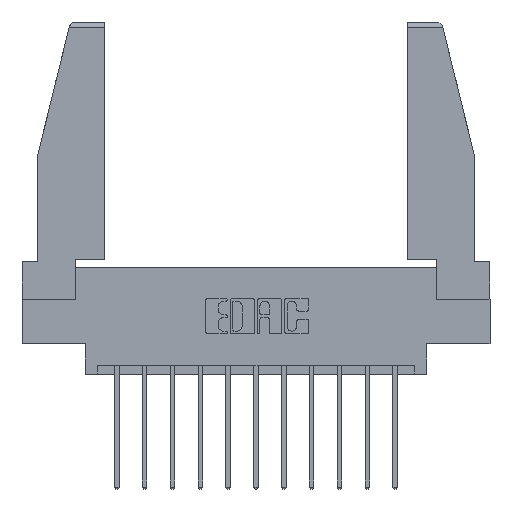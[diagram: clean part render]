
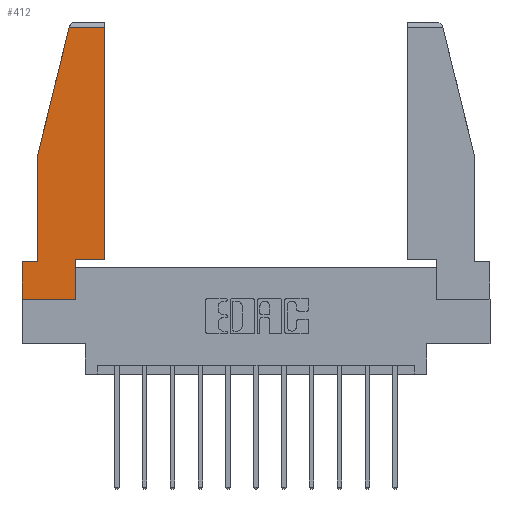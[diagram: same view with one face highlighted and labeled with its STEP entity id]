
A CAD part, top view. The second image highlights one B-rep face of the part: STEP entity #412.
In plain terms, the highlighted planar face has unit normal (0, 0, 1).
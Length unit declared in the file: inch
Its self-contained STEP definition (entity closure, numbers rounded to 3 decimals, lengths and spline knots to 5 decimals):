
#412 = ADVANCED_FACE ( 'NONE', ( #4987 ), #615, .T. ) ;
#585 = EDGE_CURVE ( 'NONE', #11403, #2946, #2954, .T. ) ;
#615 = PLANE ( 'NONE',  #14132 ) ;
#781 = VERTEX_POINT ( 'NONE', #3875 ) ;
#882 = CARTESIAN_POINT ( 'NONE',  ( 0.297, 0., 0. ) ) ;
#1013 = ORIENTED_EDGE ( 'NONE', *, *, #5995, .T. ) ;
#1213 = LINE ( 'NONE', #9749, #13338 ) ;
#1248 = LINE ( 'NONE', #13037, #14438 ) ;
#1389 = DIRECTION ( 'NONE',  ( 1., 0., 0. ) ) ;
#1553 = EDGE_CURVE ( 'NONE', #7797, #781, #8787, .T. ) ;
#1920 = CARTESIAN_POINT ( 'NONE',  ( 0.271, 1.55, 0. ) ) ;
#2297 = DIRECTION ( 'NONE',  ( 0., 1., 0. ) ) ;
#2397 = ORIENTED_EDGE ( 'NONE', *, *, #3390, .T. ) ;
#2586 = VECTOR ( 'NONE', #1389, 39.37008 ) ;
#2946 = VERTEX_POINT ( 'NONE', #5518 ) ;
#2954 = LINE ( 'NONE', #7276, #2586 ) ;
#2974 = DIRECTION ( 'NONE',  ( -0.239, -0.971, 0. ) ) ;
#3390 = EDGE_CURVE ( 'NONE', #13876, #11403, #7175, .T. ) ;
#3395 = VECTOR ( 'NONE', #9940, 39.37008 ) ;
#3468 = CARTESIAN_POINT ( 'NONE',  ( 0., 0., 0. ) ) ;
#3744 = EDGE_CURVE ( 'NONE', #781, #8341, #7984, .T. ) ;
#3875 = CARTESIAN_POINT ( 'NONE',  ( 0.086, 0.8, 0. ) ) ;
#3936 = LINE ( 'NONE', #5232, #12155 ) ;
#4003 = EDGE_CURVE ( 'NONE', #2946, #7961, #9413, .T. ) ;
#4074 = CARTESIAN_POINT ( 'NONE',  ( 0.086, 0.8, 0. ) ) ;
#4255 = CARTESIAN_POINT ( 'NONE',  ( 0., 0., 0. ) ) ;
#4987 = FACE_OUTER_BOUND ( 'NONE', #12241, .T. ) ;
#5231 = ORIENTED_EDGE ( 'NONE', *, *, #1553, .T. ) ;
#5232 = CARTESIAN_POINT ( 'NONE',  ( 0., 1.52, 0. ) ) ;
#5275 = DIRECTION ( 'NONE',  ( 1., 0., 0. ) ) ;
#5518 = CARTESIAN_POINT ( 'NONE',  ( 0.461, 0.223, 0. ) ) ;
#5841 = CARTESIAN_POINT ( 'NONE',  ( 0.297, 0.223, 0. ) ) ;
#5995 = EDGE_CURVE ( 'NONE', #8341, #9456, #1248, .T. ) ;
#6191 = ORIENTED_EDGE ( 'NONE', *, *, #4003, .T. ) ;
#6343 = CARTESIAN_POINT ( 'NONE',  ( 0., 0., 0. ) ) ;
#6649 = DIRECTION ( 'NONE',  ( 0., 1., 0. ) ) ;
#7175 = LINE ( 'NONE', #882, #9466 ) ;
#7276 = CARTESIAN_POINT ( 'NONE',  ( 0.297, 0.223, 0. ) ) ;
#7795 = DIRECTION ( 'NONE',  ( 1., 0., 0. ) ) ;
#7797 = VERTEX_POINT ( 'NONE', #11189 ) ;
#7961 = VERTEX_POINT ( 'NONE', #13493 ) ;
#7984 = LINE ( 'NONE', #4074, #3395 ) ;
#8187 = ORIENTED_EDGE ( 'NONE', *, *, #9567, .T. ) ;
#8341 = VERTEX_POINT ( 'NONE', #11113 ) ;
#8418 = ORIENTED_EDGE ( 'NONE', *, *, #3744, .T. ) ;
#8441 = DIRECTION ( 'NONE',  ( 0., -1., 0. ) ) ;
#8645 = ORIENTED_EDGE ( 'NONE', *, *, #585, .T. ) ;
#8787 = LINE ( 'NONE', #1920, #13576 ) ;
#9253 = CARTESIAN_POINT ( 'NONE',  ( 0.461, 0.223, 0. ) ) ;
#9347 = EDGE_CURVE ( 'NONE', #9456, #11376, #1213, .T. ) ;
#9413 = LINE ( 'NONE', #9253, #15070 ) ;
#9456 = VERTEX_POINT ( 'NONE', #10641 ) ;
#9466 = VECTOR ( 'NONE', #6649, 39.37008 ) ;
#9567 = EDGE_CURVE ( 'NONE', #7961, #7797, #3936, .T. ) ;
#9711 = VECTOR ( 'NONE', #5275, 39.37008 ) ;
#9749 = CARTESIAN_POINT ( 'NONE',  ( 0., 0.21, 0. ) ) ;
#9940 = DIRECTION ( 'NONE',  ( 0., -1., 0. ) ) ;
#10641 = CARTESIAN_POINT ( 'NONE',  ( 0., 0.21, 0. ) ) ;
#10754 = ORIENTED_EDGE ( 'NONE', *, *, #9347, .T. ) ;
#11113 = CARTESIAN_POINT ( 'NONE',  ( 0.086, 0.21, 0. ) ) ;
#11189 = CARTESIAN_POINT ( 'NONE',  ( 0.2636, 1.52, 0. ) ) ;
#11339 = ORIENTED_EDGE ( 'NONE', *, *, #13700, .T. ) ;
#11376 = VERTEX_POINT ( 'NONE', #3468 ) ;
#11403 = VERTEX_POINT ( 'NONE', #5841 ) ;
#11758 = DIRECTION ( 'NONE',  ( -1., 0., 0. ) ) ;
#12155 = VECTOR ( 'NONE', #12244, 39.37008 ) ;
#12241 = EDGE_LOOP ( 'NONE', ( #6191, #8187, #5231, #8418, #1013, #10754, #11339, #2397, #8645 ) ) ;
#12244 = DIRECTION ( 'NONE',  ( -1., 0., 0. ) ) ;
#12425 = DIRECTION ( 'NONE',  ( 0., 0., 1. ) ) ;
#13037 = CARTESIAN_POINT ( 'NONE',  ( 0., 0.21, 0. ) ) ;
#13338 = VECTOR ( 'NONE', #8441, 39.37008 ) ;
#13493 = CARTESIAN_POINT ( 'NONE',  ( 0.461, 1.52, 0. ) ) ;
#13576 = VECTOR ( 'NONE', #2974, 39.37008 ) ;
#13600 = CARTESIAN_POINT ( 'NONE',  ( 0.297, 0., 0. ) ) ;
#13700 = EDGE_CURVE ( 'NONE', #11376, #13876, #13982, .T. ) ;
#13876 = VERTEX_POINT ( 'NONE', #13600 ) ;
#13982 = LINE ( 'NONE', #6343, #9711 ) ;
#14132 = AXIS2_PLACEMENT_3D ( 'NONE', #4255, #12425, #7795 ) ;
#14438 = VECTOR ( 'NONE', #11758, 39.37008 ) ;
#15070 = VECTOR ( 'NONE', #2297, 39.37008 ) ;
